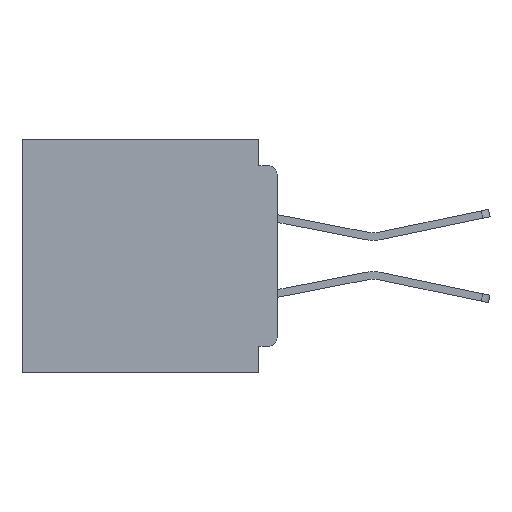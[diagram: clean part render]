
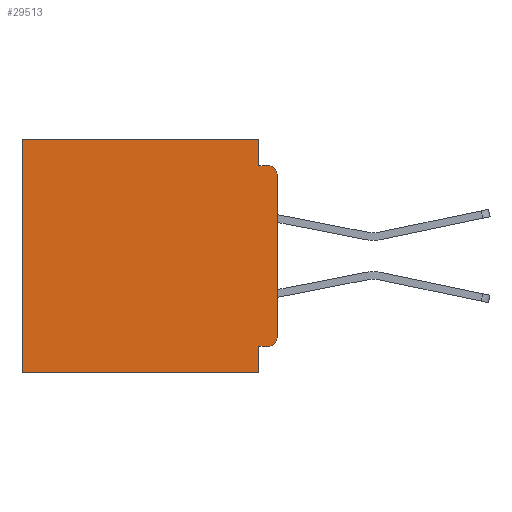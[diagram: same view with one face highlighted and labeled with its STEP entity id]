
A CAD part, left-side view. The second image highlights one B-rep face of the part: STEP entity #29513.
In plain terms, the highlighted planar face has unit normal (-1, 0, 0).
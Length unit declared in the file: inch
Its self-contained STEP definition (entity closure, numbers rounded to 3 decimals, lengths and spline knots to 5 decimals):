
#1067 = AXIS2_PLACEMENT_3D ( 'NONE', #26829, #7682, #41410 ) ;
#1379 = LINE ( 'NONE', #2702, #11279 ) ;
#1815 = LINE ( 'NONE', #50647, #13192 ) ;
#2434 = VERTEX_POINT ( 'NONE', #29079 ) ;
#2702 = CARTESIAN_POINT ( 'NONE',  ( 0.3, 0., 0. ) ) ;
#3653 = CARTESIAN_POINT ( 'NONE',  ( 0.3, 0.437, -0.4 ) ) ;
#3728 = VECTOR ( 'NONE', #49007, 39.37008 ) ;
#4671 = LINE ( 'NONE', #18629, #41655 ) ;
#4965 = FACE_OUTER_BOUND ( 'NONE', #7163, .T. ) ;
#4995 = ORIENTED_EDGE ( 'NONE', *, *, #60719, .T. ) ;
#5168 = CARTESIAN_POINT ( 'NONE',  ( 0.3, 0., -0.355 ) ) ;
#5293 = CARTESIAN_POINT ( 'NONE',  ( 0.3, 0.015, -0.045 ) ) ;
#5304 = DIRECTION ( 'NONE',  ( -1., 0., 0. ) ) ;
#7024 = VERTEX_POINT ( 'NONE', #59991 ) ;
#7163 = EDGE_LOOP ( 'NONE', ( #34027, #4995, #54928, #51399, #15490, #22328, #42409, #59340, #18218, #48022 ) ) ;
#7268 = CARTESIAN_POINT ( 'NONE',  ( 0.3, 0., -0.4 ) ) ;
#7611 = DIRECTION ( 'NONE',  ( 0., 1., 0. ) ) ;
#7682 = DIRECTION ( 'NONE',  ( 1., 0., 0. ) ) ;
#10696 = LINE ( 'NONE', #19099, #49149 ) ;
#11279 = VECTOR ( 'NONE', #7611, 39.37008 ) ;
#11394 = CARTESIAN_POINT ( 'NONE',  ( 0.3, 0.015, -0.06 ) ) ;
#12091 = DIRECTION ( 'NONE',  ( 0., 1., 0. ) ) ;
#12888 = LINE ( 'NONE', #5168, #61129 ) ;
#13192 = VECTOR ( 'NONE', #21791, 39.37008 ) ;
#13283 = CIRCLE ( 'NONE', #18164, 0.015 ) ;
#14630 = DIRECTION ( 'NONE',  ( 0., 0., -1. ) ) ;
#14894 = DIRECTION ( 'NONE',  ( 0., 1., 0. ) ) ;
#15490 = ORIENTED_EDGE ( 'NONE', *, *, #51616, .T. ) ;
#16258 = DIRECTION ( 'NONE',  ( 0., 0., -1. ) ) ;
#16711 = VERTEX_POINT ( 'NONE', #3653 ) ;
#17145 = EDGE_CURVE ( 'NONE', #7024, #16711, #41860, .T. ) ;
#17181 = EDGE_CURVE ( 'NONE', #2434, #7024, #1815, .T. ) ;
#18164 = AXIS2_PLACEMENT_3D ( 'NONE', #34233, #5304, #39063 ) ;
#18218 = ORIENTED_EDGE ( 'NONE', *, *, #50711, .F. ) ;
#18629 = CARTESIAN_POINT ( 'NONE',  ( 0.3, 0., -0.045 ) ) ;
#19099 = CARTESIAN_POINT ( 'NONE',  ( 0.3, 0.031, 0. ) ) ;
#19219 = VERTEX_POINT ( 'NONE', #47487 ) ;
#20569 = VERTEX_POINT ( 'NONE', #38308 ) ;
#20715 = EDGE_CURVE ( 'NONE', #32783, #16711, #27860, .T. ) ;
#21791 = DIRECTION ( 'NONE',  ( 0., 0., -1. ) ) ;
#22328 = ORIENTED_EDGE ( 'NONE', *, *, #20715, .T. ) ;
#23448 = DIRECTION ( 'NONE',  ( 0., -1., 0. ) ) ;
#26829 = CARTESIAN_POINT ( 'NONE',  ( 0.3, 0., -0.4 ) ) ;
#27860 = LINE ( 'NONE', #29629, #3728 ) ;
#29079 = CARTESIAN_POINT ( 'NONE',  ( 0.3, 0.031, -0.355 ) ) ;
#29513 = ADVANCED_FACE ( 'NONE', ( #4965 ), #31701, .F. ) ;
#29629 = CARTESIAN_POINT ( 'NONE',  ( 0.3, 0.437, -0.4 ) ) ;
#30435 = CIRCLE ( 'NONE', #30472, 0.015 ) ;
#30472 = AXIS2_PLACEMENT_3D ( 'NONE', #11394, #45105, #16258 ) ;
#31701 = PLANE ( 'NONE',  #1067 ) ;
#32770 = EDGE_CURVE ( 'NONE', #19219, #35222, #10696, .T. ) ;
#32783 = VERTEX_POINT ( 'NONE', #33632 ) ;
#32812 = LINE ( 'NONE', #43515, #58441 ) ;
#33632 = CARTESIAN_POINT ( 'NONE',  ( 0.3, 0.437, 0. ) ) ;
#34027 = ORIENTED_EDGE ( 'NONE', *, *, #60008, .F. ) ;
#34233 = CARTESIAN_POINT ( 'NONE',  ( 0.3, 0.015, -0.34 ) ) ;
#35222 = VERTEX_POINT ( 'NONE', #61368 ) ;
#37677 = VERTEX_POINT ( 'NONE', #5293 ) ;
#38308 = CARTESIAN_POINT ( 'NONE',  ( 0.3, 0., -0.34 ) ) ;
#39063 = DIRECTION ( 'NONE',  ( 0., 0., -1. ) ) ;
#40081 = EDGE_CURVE ( 'NONE', #60092, #20569, #13283, .T. ) ;
#41410 = DIRECTION ( 'NONE',  ( 0., 0., -1. ) ) ;
#41655 = VECTOR ( 'NONE', #23448, 39.37008 ) ;
#41860 = LINE ( 'NONE', #7268, #51650 ) ;
#42409 = ORIENTED_EDGE ( 'NONE', *, *, #17145, .F. ) ;
#43515 = CARTESIAN_POINT ( 'NONE',  ( 0.3, 0., -0.4 ) ) ;
#45105 = DIRECTION ( 'NONE',  ( -1., 0., 0. ) ) ;
#47487 = CARTESIAN_POINT ( 'NONE',  ( 0.3, 0.031, 0. ) ) ;
#48022 = ORIENTED_EDGE ( 'NONE', *, *, #40081, .T. ) ;
#49007 = DIRECTION ( 'NONE',  ( 0., 0., -1. ) ) ;
#49149 = VECTOR ( 'NONE', #57636, 39.37008 ) ;
#50647 = CARTESIAN_POINT ( 'NONE',  ( 0.3, 0.031, -0.4 ) ) ;
#50711 = EDGE_CURVE ( 'NONE', #60092, #2434, #12888, .T. ) ;
#51399 = ORIENTED_EDGE ( 'NONE', *, *, #32770, .F. ) ;
#51616 = EDGE_CURVE ( 'NONE', #19219, #32783, #1379, .T. ) ;
#51650 = VECTOR ( 'NONE', #12091, 39.37008 ) ;
#53589 = CARTESIAN_POINT ( 'NONE',  ( 0.3, 0.015, -0.355 ) ) ;
#54928 = ORIENTED_EDGE ( 'NONE', *, *, #57439, .F. ) ;
#57439 = EDGE_CURVE ( 'NONE', #35222, #37677, #4671, .T. ) ;
#57636 = DIRECTION ( 'NONE',  ( 0., 0., -1. ) ) ;
#58441 = VECTOR ( 'NONE', #14630, 39.37008 ) ;
#58892 = CARTESIAN_POINT ( 'NONE',  ( 0.3, 0., -0.06 ) ) ;
#58961 = VERTEX_POINT ( 'NONE', #58892 ) ;
#59340 = ORIENTED_EDGE ( 'NONE', *, *, #17181, .F. ) ;
#59991 = CARTESIAN_POINT ( 'NONE',  ( 0.3, 0.031, -0.4 ) ) ;
#60008 = EDGE_CURVE ( 'NONE', #58961, #20569, #32812, .T. ) ;
#60092 = VERTEX_POINT ( 'NONE', #53589 ) ;
#60719 = EDGE_CURVE ( 'NONE', #58961, #37677, #30435, .T. ) ;
#61129 = VECTOR ( 'NONE', #14894, 39.37008 ) ;
#61368 = CARTESIAN_POINT ( 'NONE',  ( 0.3, 0.031, -0.045 ) ) ;
